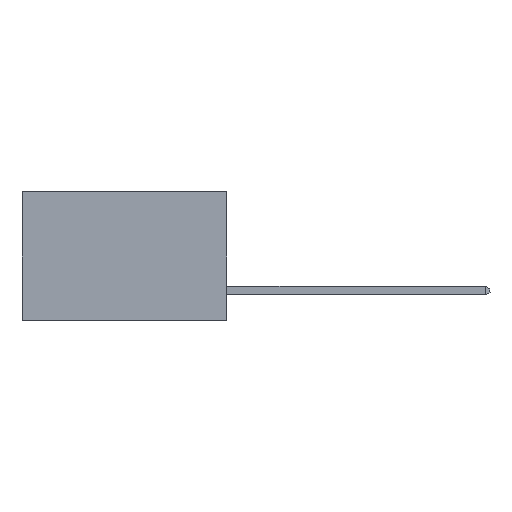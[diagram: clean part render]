
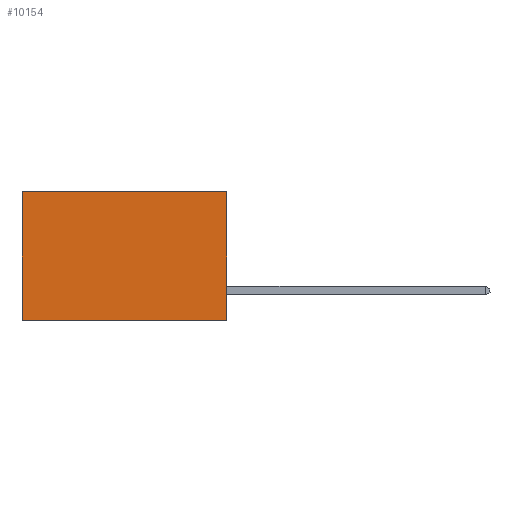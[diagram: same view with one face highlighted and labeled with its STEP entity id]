
A CAD part, left-side view. The second image highlights one B-rep face of the part: STEP entity #10154.
In plain terms, the highlighted planar face has unit normal (-1, 0, 0).
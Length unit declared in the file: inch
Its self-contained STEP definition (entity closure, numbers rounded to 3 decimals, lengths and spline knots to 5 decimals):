
#310 = CARTESIAN_POINT ( 'NONE',  ( 0.277, 0., -0.37 ) ) ;
#423 = VERTEX_POINT ( 'NONE', #4887 ) ;
#613 = CARTESIAN_POINT ( 'NONE',  ( 0.277, 0., -0.37 ) ) ;
#1041 = PLANE ( 'NONE',  #10216 ) ;
#1122 = EDGE_LOOP ( 'NONE', ( #7691, #7730, #7991, #8296 ) ) ;
#1690 = EDGE_CURVE ( 'NONE', #423, #5224, #4246, .T. ) ;
#1738 = FACE_OUTER_BOUND ( 'NONE', #1122, .T. ) ;
#1827 = VECTOR ( 'NONE', #3025, 39.37008 ) ;
#1835 = DIRECTION ( 'NONE',  ( 0., 0., -1. ) ) ;
#2172 = VERTEX_POINT ( 'NONE', #2676 ) ;
#2241 = LINE ( 'NONE', #8006, #10112 ) ;
#2315 = DIRECTION ( 'NONE',  ( 0., 1., 0. ) ) ;
#2633 = EDGE_CURVE ( 'NONE', #8478, #2172, #6943, .T. ) ;
#2672 = EDGE_CURVE ( 'NONE', #423, #8478, #8455, .T. ) ;
#2676 = CARTESIAN_POINT ( 'NONE',  ( 0.277, 0.59, -0.37 ) ) ;
#2745 = CARTESIAN_POINT ( 'NONE',  ( 0.277, 0., 0. ) ) ;
#3025 = DIRECTION ( 'NONE',  ( 0., 0., -1. ) ) ;
#3115 = CARTESIAN_POINT ( 'NONE',  ( 0.277, 0.59, -0.37 ) ) ;
#3792 = DIRECTION ( 'NONE',  ( 1., 0., 0. ) ) ;
#4246 = LINE ( 'NONE', #310, #1827 ) ;
#4377 = VECTOR ( 'NONE', #6085, 39.37008 ) ;
#4887 = CARTESIAN_POINT ( 'NONE',  ( 0.277, 0., 0. ) ) ;
#5133 = VECTOR ( 'NONE', #1835, 39.37008 ) ;
#5224 = VERTEX_POINT ( 'NONE', #613 ) ;
#6085 = DIRECTION ( 'NONE',  ( 0., 1., 0. ) ) ;
#6943 = LINE ( 'NONE', #3115, #5133 ) ;
#7618 = CARTESIAN_POINT ( 'NONE',  ( 0.277, 0.59, 0. ) ) ;
#7691 = ORIENTED_EDGE ( 'NONE', *, *, #2633, .T. ) ;
#7730 = ORIENTED_EDGE ( 'NONE', *, *, #7998, .F. ) ;
#7991 = ORIENTED_EDGE ( 'NONE', *, *, #1690, .F. ) ;
#7998 = EDGE_CURVE ( 'NONE', #5224, #2172, #2241, .T. ) ;
#8006 = CARTESIAN_POINT ( 'NONE',  ( 0.277, 0., -0.37 ) ) ;
#8296 = ORIENTED_EDGE ( 'NONE', *, *, #2672, .T. ) ;
#8455 = LINE ( 'NONE', #2745, #4377 ) ;
#8478 = VERTEX_POINT ( 'NONE', #7618 ) ;
#8479 = CARTESIAN_POINT ( 'NONE',  ( 0.277, 0., -0.37 ) ) ;
#9228 = DIRECTION ( 'NONE',  ( 0., 0., -1. ) ) ;
#10112 = VECTOR ( 'NONE', #2315, 39.37008 ) ;
#10154 = ADVANCED_FACE ( 'NONE', ( #1738 ), #1041, .F. ) ;
#10216 = AXIS2_PLACEMENT_3D ( 'NONE', #8479, #3792, #9228 ) ;
